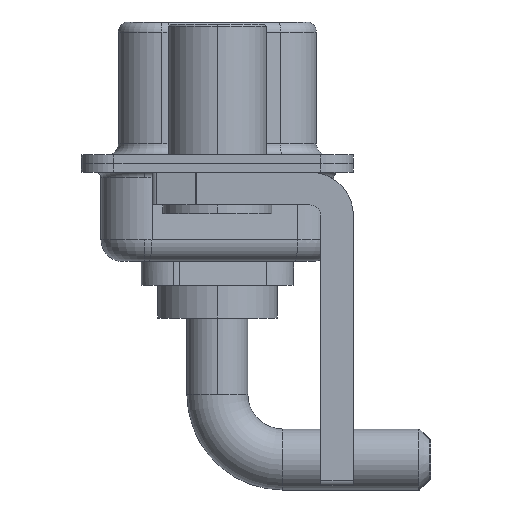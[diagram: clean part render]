
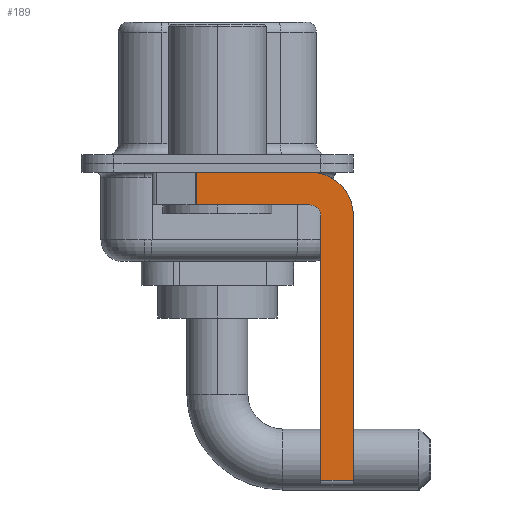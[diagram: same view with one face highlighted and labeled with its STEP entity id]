
A CAD part, left-side view. The second image highlights one B-rep face of the part: STEP entity #189.
In plain terms, the highlighted planar face has unit normal (-1, 0, 0).
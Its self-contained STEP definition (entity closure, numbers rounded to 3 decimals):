
#22 = CARTESIAN_POINT ( 'NONE',  ( -2.9, -6.25, -2.4 ) ) ;
#180 = VERTEX_POINT ( 'NONE', #14641 ) ;
#189 = ADVANCED_FACE ( 'NONE', ( #13353 ), #1664, .F. ) ;
#243 = VERTEX_POINT ( 'NONE', #2245 ) ;
#711 = LINE ( 'NONE', #4478, #5692 ) ;
#721 = DIRECTION ( 'NONE',  ( 0., 0., -1. ) ) ;
#866 = EDGE_CURVE ( 'NONE', #4523, #3812, #15534, .T. ) ;
#1415 = CIRCLE ( 'NONE', #5526, 0.5 ) ;
#1644 = VERTEX_POINT ( 'NONE', #4903 ) ;
#1664 = PLANE ( 'NONE',  #15110 ) ;
#1915 = EDGE_CURVE ( 'NONE', #243, #1644, #711, .T. ) ;
#1944 = ORIENTED_EDGE ( 'NONE', *, *, #2739, .F. ) ;
#1980 = DIRECTION ( 'NONE',  ( 1., 0., 0. ) ) ;
#2245 = CARTESIAN_POINT ( 'NONE',  ( -2.9, 0.978, -0.4 ) ) ;
#2739 = EDGE_CURVE ( 'NONE', #6944, #9527, #1415, .T. ) ;
#3095 = DIRECTION ( 'NONE',  ( 0., 0., -1. ) ) ;
#3326 = VECTOR ( 'NONE', #11460, 1000. ) ;
#3812 = VERTEX_POINT ( 'NONE', #10921 ) ;
#3849 = ORIENTED_EDGE ( 'NONE', *, *, #10291, .F. ) ;
#3946 = ORIENTED_EDGE ( 'NONE', *, *, #8001, .T. ) ;
#4476 = DIRECTION ( 'NONE',  ( 0., 0., 1. ) ) ;
#4478 = CARTESIAN_POINT ( 'NONE',  ( -2.9, 0.978, -1.9 ) ) ;
#4515 = CARTESIAN_POINT ( 'NONE',  ( -2.9, -4.75, -2.4 ) ) ;
#4523 = VERTEX_POINT ( 'NONE', #22 ) ;
#4640 = DIRECTION ( 'NONE',  ( 1., 0., 0. ) ) ;
#4684 = CIRCLE ( 'NONE', #13674, 2. ) ;
#4903 = CARTESIAN_POINT ( 'NONE',  ( -2.9, 0.978, -1.9 ) ) ;
#5526 = AXIS2_PLACEMENT_3D ( 'NONE', #6785, #16154, #4476 ) ;
#5692 = VECTOR ( 'NONE', #3095, 1000. ) ;
#6527 = EDGE_CURVE ( 'NONE', #180, #4523, #4684, .T. ) ;
#6540 = LINE ( 'NONE', #14305, #12906 ) ;
#6610 = EDGE_LOOP ( 'NONE', ( #12404, #14128, #8221, #1944, #3849, #3946, #7185, #10201 ) ) ;
#6627 = DIRECTION ( 'NONE',  ( 0., 1., 0. ) ) ;
#6785 = CARTESIAN_POINT ( 'NONE',  ( -2.9, -4.25, -2.4 ) ) ;
#6944 = VERTEX_POINT ( 'NONE', #4515 ) ;
#7122 = DIRECTION ( 'NONE',  ( 0., -1., 0. ) ) ;
#7185 = ORIENTED_EDGE ( 'NONE', *, *, #866, .F. ) ;
#7193 = VECTOR ( 'NONE', #15713, 1000. ) ;
#7338 = LINE ( 'NONE', #12696, #9407 ) ;
#7516 = DIRECTION ( 'NONE',  ( 0., 0., 1. ) ) ;
#7565 = CARTESIAN_POINT ( 'NONE',  ( -2.9, -4.75, -14.55 ) ) ;
#7772 = CARTESIAN_POINT ( 'NONE',  ( -2.9, -4.25, -1.9 ) ) ;
#7806 = CARTESIAN_POINT ( 'NONE',  ( -2.9, -6.25, -2.4 ) ) ;
#8001 = EDGE_CURVE ( 'NONE', #14695, #3812, #12546, .T. ) ;
#8221 = ORIENTED_EDGE ( 'NONE', *, *, #14084, .F. ) ;
#9407 = VECTOR ( 'NONE', #7516, 1000. ) ;
#9527 = VERTEX_POINT ( 'NONE', #7772 ) ;
#10201 = ORIENTED_EDGE ( 'NONE', *, *, #6527, .F. ) ;
#10291 = EDGE_CURVE ( 'NONE', #14695, #6944, #7338, .T. ) ;
#10921 = CARTESIAN_POINT ( 'NONE',  ( -2.9, -6.25, -14.55 ) ) ;
#11192 = DIRECTION ( 'NONE',  ( 0., 0., -1. ) ) ;
#11293 = CARTESIAN_POINT ( 'NONE',  ( -2.9, -4.25, -14.55 ) ) ;
#11460 = DIRECTION ( 'NONE',  ( 0., -1., 0. ) ) ;
#12404 = ORIENTED_EDGE ( 'NONE', *, *, #12767, .F. ) ;
#12546 = LINE ( 'NONE', #11293, #13719 ) ;
#12696 = CARTESIAN_POINT ( 'NONE',  ( -2.9, -4.75, -14.8 ) ) ;
#12767 = EDGE_CURVE ( 'NONE', #243, #180, #15212, .T. ) ;
#12906 = VECTOR ( 'NONE', #6627, 1000. ) ;
#13353 = FACE_OUTER_BOUND ( 'NONE', #6610, .T. ) ;
#13674 = AXIS2_PLACEMENT_3D ( 'NONE', #16313, #1980, #11192 ) ;
#13719 = VECTOR ( 'NONE', #7122, 1000. ) ;
#14084 = EDGE_CURVE ( 'NONE', #9527, #1644, #6540, .T. ) ;
#14128 = ORIENTED_EDGE ( 'NONE', *, *, #1915, .T. ) ;
#14190 = CARTESIAN_POINT ( 'NONE',  ( -2.9, 3., -0.4 ) ) ;
#14305 = CARTESIAN_POINT ( 'NONE',  ( -2.9, -4.25, -1.9 ) ) ;
#14641 = CARTESIAN_POINT ( 'NONE',  ( -2.9, -4.25, -0.4 ) ) ;
#14695 = VERTEX_POINT ( 'NONE', #7565 ) ;
#15110 = AXIS2_PLACEMENT_3D ( 'NONE', #15213, #4640, #721 ) ;
#15212 = LINE ( 'NONE', #14190, #3326 ) ;
#15213 = CARTESIAN_POINT ( 'NONE',  ( -2.9, -4.25, -2.4 ) ) ;
#15534 = LINE ( 'NONE', #7806, #7193 ) ;
#15713 = DIRECTION ( 'NONE',  ( 0., 0., -1. ) ) ;
#16154 = DIRECTION ( 'NONE',  ( -1., 0., 0. ) ) ;
#16313 = CARTESIAN_POINT ( 'NONE',  ( -2.9, -4.25, -2.4 ) ) ;
